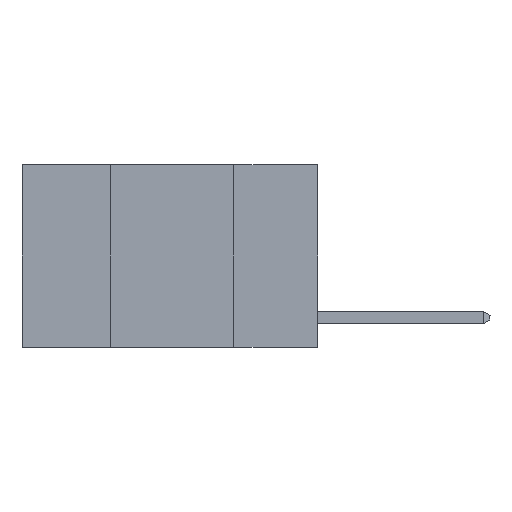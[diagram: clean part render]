
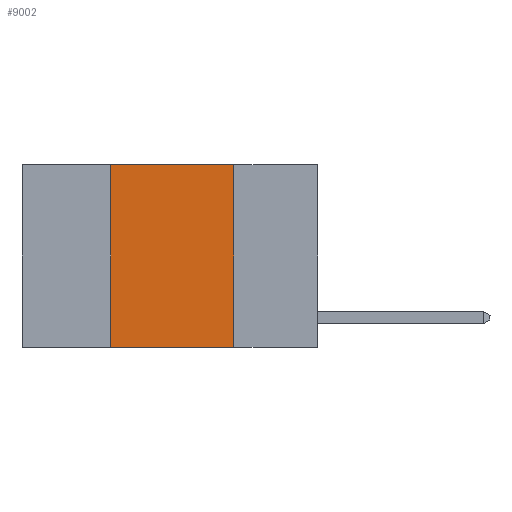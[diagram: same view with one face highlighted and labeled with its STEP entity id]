
A CAD part, left-side view. The second image highlights one B-rep face of the part: STEP entity #9002.
In plain terms, the highlighted planar face has unit normal (-1, 0, 0).
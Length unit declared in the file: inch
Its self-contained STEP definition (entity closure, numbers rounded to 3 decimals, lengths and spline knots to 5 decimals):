
#362 = FACE_OUTER_BOUND ( 'NONE', #24189, .T. ) ;
#1153 = DIRECTION ( 'NONE',  ( 0., 0., -1. ) ) ;
#1327 = DIRECTION ( 'NONE',  ( 0., -1., 0. ) ) ;
#1394 = EDGE_CURVE ( 'NONE', #28383, #19079, #5769, .T. ) ;
#3428 = VERTEX_POINT ( 'NONE', #12307 ) ;
#3821 = DIRECTION ( 'NONE',  ( 0., -1., 0. ) ) ;
#4622 = LINE ( 'NONE', #15761, #5124 ) ;
#4965 = CARTESIAN_POINT ( 'NONE',  ( 0., 0.6, 0. ) ) ;
#5124 = VECTOR ( 'NONE', #22747, 39.37008 ) ;
#5685 = VECTOR ( 'NONE', #1153, 39.37008 ) ;
#5769 = LINE ( 'NONE', #8450, #23658 ) ;
#6752 = DIRECTION ( 'NONE',  ( 0., 0., -1. ) ) ;
#7096 = LINE ( 'NONE', #16169, #5685 ) ;
#8450 = CARTESIAN_POINT ( 'NONE',  ( 0., 0.6, 0. ) ) ;
#8455 = VERTEX_POINT ( 'NONE', #27881 ) ;
#9002 = ADVANCED_FACE ( 'NONE', ( #362 ), #25323, .F. ) ;
#9371 = VECTOR ( 'NONE', #3821, 39.37008 ) ;
#9753 = CARTESIAN_POINT ( 'NONE',  ( 0., 0.42, 0. ) ) ;
#12307 = CARTESIAN_POINT ( 'NONE',  ( 0., 0.42, -0.37 ) ) ;
#13464 = ORIENTED_EDGE ( 'NONE', *, *, #24170, .T. ) ;
#14435 = ORIENTED_EDGE ( 'NONE', *, *, #28358, .F. ) ;
#15091 = LINE ( 'NONE', #17171, #9371 ) ;
#15761 = CARTESIAN_POINT ( 'NONE',  ( 0., 0.42, 0. ) ) ;
#16169 = CARTESIAN_POINT ( 'NONE',  ( 0., 0.17, 0. ) ) ;
#16423 = CARTESIAN_POINT ( 'NONE',  ( 0., 0.17, 0. ) ) ;
#17171 = CARTESIAN_POINT ( 'NONE',  ( 0., 0.6, -0.37 ) ) ;
#18043 = DIRECTION ( 'NONE',  ( 1., 0., 0. ) ) ;
#19079 = VERTEX_POINT ( 'NONE', #16423 ) ;
#22747 = DIRECTION ( 'NONE',  ( 0., 0., 1. ) ) ;
#23658 = VECTOR ( 'NONE', #1327, 39.37008 ) ;
#24170 = EDGE_CURVE ( 'NONE', #3428, #8455, #15091, .T. ) ;
#24189 = EDGE_LOOP ( 'NONE', ( #14435, #26491, #26999, #13464 ) ) ;
#24865 = AXIS2_PLACEMENT_3D ( 'NONE', #4965, #18043, #6752 ) ;
#25323 = PLANE ( 'NONE',  #24865 ) ;
#26491 = ORIENTED_EDGE ( 'NONE', *, *, #1394, .F. ) ;
#26684 = EDGE_CURVE ( 'NONE', #3428, #28383, #4622, .T. ) ;
#26999 = ORIENTED_EDGE ( 'NONE', *, *, #26684, .F. ) ;
#27881 = CARTESIAN_POINT ( 'NONE',  ( 0., 0.17, -0.37 ) ) ;
#28358 = EDGE_CURVE ( 'NONE', #19079, #8455, #7096, .T. ) ;
#28383 = VERTEX_POINT ( 'NONE', #9753 ) ;
